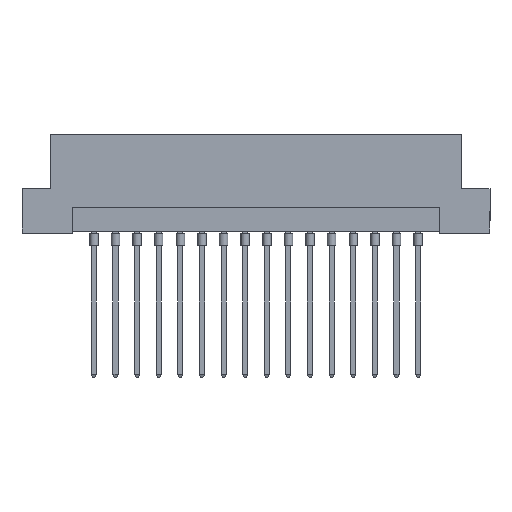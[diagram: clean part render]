
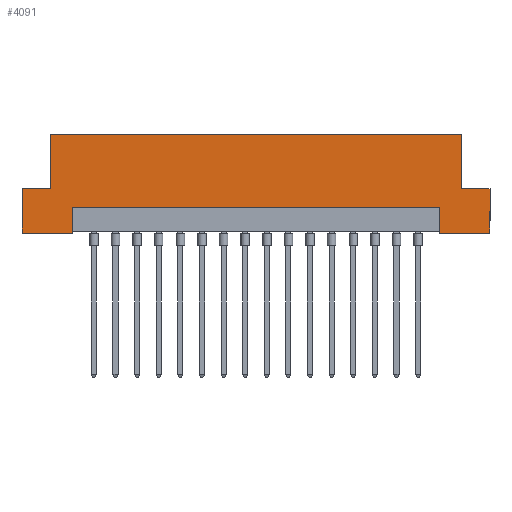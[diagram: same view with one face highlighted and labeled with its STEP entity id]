
A CAD part, front view. The second image highlights one B-rep face of the part: STEP entity #4091.
In plain terms, the highlighted planar face has unit normal (0, -1, 0).
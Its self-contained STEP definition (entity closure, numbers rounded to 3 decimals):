
#2 = CARTESIAN_POINT ( 'NONE',  ( -21.6, -4.3, 3. ) ) ;
#103 = PLANE ( 'NONE',  #130 ) ;
#130 = AXIS2_PLACEMENT_3D ( 'NONE', #2309, #6668, #549 ) ;
#206 = VECTOR ( 'NONE', #3185, 1000. ) ;
#326 = DIRECTION ( 'NONE',  ( 0., 0., -1. ) ) ;
#549 = DIRECTION ( 'NONE',  ( -1., 0., 0. ) ) ;
#552 = LINE ( 'NONE', #2, #6739 ) ;
#557 = CARTESIAN_POINT ( 'NONE',  ( -27.5, -4.3, 5.2 ) ) ;
#579 = ORIENTED_EDGE ( 'NONE', *, *, #829, .F. ) ;
#670 = VERTEX_POINT ( 'NONE', #2685 ) ;
#740 = ORIENTED_EDGE ( 'NONE', *, *, #3811, .T. ) ;
#774 = ORIENTED_EDGE ( 'NONE', *, *, #5839, .T. ) ;
#792 = VERTEX_POINT ( 'NONE', #2486 ) ;
#829 = EDGE_CURVE ( 'NONE', #3084, #792, #4149, .T. ) ;
#835 = CARTESIAN_POINT ( 'NONE',  ( 27.5, -4.3, 11.6 ) ) ;
#889 = ORIENTED_EDGE ( 'NONE', *, *, #3107, .F. ) ;
#1007 = CARTESIAN_POINT ( 'NONE',  ( 24.2, -4.3, 11.6 ) ) ;
#1093 = VECTOR ( 'NONE', #326, 1000. ) ;
#1179 = CARTESIAN_POINT ( 'NONE',  ( -24.2, -4.3, 11.6 ) ) ;
#1221 = VERTEX_POINT ( 'NONE', #3949 ) ;
#1321 = EDGE_CURVE ( 'NONE', #4698, #2654, #3849, .T. ) ;
#1358 = EDGE_CURVE ( 'NONE', #4435, #5169, #5413, .T. ) ;
#1400 = ORIENTED_EDGE ( 'NONE', *, *, #6419, .F. ) ;
#1485 = LINE ( 'NONE', #1559, #2424 ) ;
#1507 = CARTESIAN_POINT ( 'NONE',  ( 24.2, -4.3, 5.2 ) ) ;
#1559 = CARTESIAN_POINT ( 'NONE',  ( -24.2, -4.3, 5.2 ) ) ;
#1581 = ORIENTED_EDGE ( 'NONE', *, *, #1358, .T. ) ;
#1678 = VECTOR ( 'NONE', #7025, 1000. ) ;
#1768 = ORIENTED_EDGE ( 'NONE', *, *, #1321, .T. ) ;
#1873 = VECTOR ( 'NONE', #6663, 1000. ) ;
#1889 = CARTESIAN_POINT ( 'NONE',  ( -27.5, -4.3, 0. ) ) ;
#1924 = VERTEX_POINT ( 'NONE', #2289 ) ;
#1949 = EDGE_LOOP ( 'NONE', ( #774, #889, #740, #579, #3532, #1768, #5623, #6495, #3735, #1581, #3248, #1400 ) ) ;
#2173 = CARTESIAN_POINT ( 'NONE',  ( 27.5, -4.3, 0. ) ) ;
#2289 = CARTESIAN_POINT ( 'NONE',  ( 21.6, -4.3, 0. ) ) ;
#2309 = CARTESIAN_POINT ( 'NONE',  ( 27.5, -4.3, 11.6 ) ) ;
#2424 = VECTOR ( 'NONE', #5394, 1000. ) ;
#2486 = CARTESIAN_POINT ( 'NONE',  ( 27.5, -4.3, 0. ) ) ;
#2616 = CARTESIAN_POINT ( 'NONE',  ( 27.5, -4.3, 5.2 ) ) ;
#2654 = VERTEX_POINT ( 'NONE', #1007 ) ;
#2670 = EDGE_CURVE ( 'NONE', #5807, #6868, #1485, .T. ) ;
#2685 = CARTESIAN_POINT ( 'NONE',  ( 21.6, -4.3, 3. ) ) ;
#2849 = CARTESIAN_POINT ( 'NONE',  ( -21.6, -4.3, 0.2 ) ) ;
#2886 = LINE ( 'NONE', #6812, #6394 ) ;
#2916 = CARTESIAN_POINT ( 'NONE',  ( 24.2, -4.3, 5.2 ) ) ;
#2957 = DIRECTION ( 'NONE',  ( 1., 0., 0. ) ) ;
#3084 = VERTEX_POINT ( 'NONE', #2616 ) ;
#3107 = EDGE_CURVE ( 'NONE', #1924, #670, #3690, .T. ) ;
#3131 = LINE ( 'NONE', #4185, #4292 ) ;
#3185 = DIRECTION ( 'NONE',  ( 0., 0., 1. ) ) ;
#3192 = DIRECTION ( 'NONE',  ( 0., 0., 1. ) ) ;
#3229 = VECTOR ( 'NONE', #3428, 1000. ) ;
#3248 = ORIENTED_EDGE ( 'NONE', *, *, #4099, .T. ) ;
#3428 = DIRECTION ( 'NONE',  ( 1., 0., 0. ) ) ;
#3499 = LINE ( 'NONE', #3564, #7079 ) ;
#3532 = ORIENTED_EDGE ( 'NONE', *, *, #6048, .F. ) ;
#3564 = CARTESIAN_POINT ( 'NONE',  ( 27.5, -4.3, 0. ) ) ;
#3608 = DIRECTION ( 'NONE',  ( 1., 0., 0. ) ) ;
#3643 = EDGE_CURVE ( 'NONE', #4435, #5807, #3837, .T. ) ;
#3690 = LINE ( 'NONE', #5442, #206 ) ;
#3735 = ORIENTED_EDGE ( 'NONE', *, *, #3643, .F. ) ;
#3811 = EDGE_CURVE ( 'NONE', #1924, #792, #3499, .T. ) ;
#3837 = LINE ( 'NONE', #557, #3229 ) ;
#3849 = LINE ( 'NONE', #1507, #5491 ) ;
#3920 = CARTESIAN_POINT ( 'NONE',  ( -21.6, -4.3, 3. ) ) ;
#3949 = CARTESIAN_POINT ( 'NONE',  ( -21.6, -4.3, 0. ) ) ;
#4091 = ADVANCED_FACE ( 'NONE', ( #4473 ), #103, .F. ) ;
#4099 = EDGE_CURVE ( 'NONE', #5169, #1221, #6057, .T. ) ;
#4149 = LINE ( 'NONE', #835, #1093 ) ;
#4185 = CARTESIAN_POINT ( 'NONE',  ( 27.5, -4.3, 11.6 ) ) ;
#4292 = VECTOR ( 'NONE', #4778, 1000. ) ;
#4435 = VERTEX_POINT ( 'NONE', #6444 ) ;
#4448 = CARTESIAN_POINT ( 'NONE',  ( -24.2, -4.3, 5.2 ) ) ;
#4473 = FACE_OUTER_BOUND ( 'NONE', #1949, .T. ) ;
#4529 = VERTEX_POINT ( 'NONE', #3920 ) ;
#4698 = VERTEX_POINT ( 'NONE', #2916 ) ;
#4749 = VECTOR ( 'NONE', #5534, 1000. ) ;
#4778 = DIRECTION ( 'NONE',  ( 1., 0., 0. ) ) ;
#5169 = VERTEX_POINT ( 'NONE', #1889 ) ;
#5394 = DIRECTION ( 'NONE',  ( 0., 0., 1. ) ) ;
#5413 = LINE ( 'NONE', #5946, #1678 ) ;
#5442 = CARTESIAN_POINT ( 'NONE',  ( 21.6, -4.3, 0.2 ) ) ;
#5491 = VECTOR ( 'NONE', #3192, 1000. ) ;
#5534 = DIRECTION ( 'NONE',  ( 1., 0., 0. ) ) ;
#5540 = DIRECTION ( 'NONE',  ( 1., 0., 0. ) ) ;
#5623 = ORIENTED_EDGE ( 'NONE', *, *, #6102, .F. ) ;
#5807 = VERTEX_POINT ( 'NONE', #4448 ) ;
#5839 = EDGE_CURVE ( 'NONE', #4529, #670, #552, .T. ) ;
#5946 = CARTESIAN_POINT ( 'NONE',  ( -27.5, -4.3, 11.6 ) ) ;
#6048 = EDGE_CURVE ( 'NONE', #4698, #3084, #2886, .T. ) ;
#6057 = LINE ( 'NONE', #2173, #4749 ) ;
#6102 = EDGE_CURVE ( 'NONE', #6868, #2654, #3131, .T. ) ;
#6163 = LINE ( 'NONE', #2849, #1873 ) ;
#6394 = VECTOR ( 'NONE', #2957, 1000. ) ;
#6419 = EDGE_CURVE ( 'NONE', #4529, #1221, #6163, .T. ) ;
#6444 = CARTESIAN_POINT ( 'NONE',  ( -27.5, -4.3, 5.2 ) ) ;
#6495 = ORIENTED_EDGE ( 'NONE', *, *, #2670, .F. ) ;
#6663 = DIRECTION ( 'NONE',  ( 0., 0., -1. ) ) ;
#6668 = DIRECTION ( 'NONE',  ( 0., 1., 0. ) ) ;
#6739 = VECTOR ( 'NONE', #5540, 1000. ) ;
#6812 = CARTESIAN_POINT ( 'NONE',  ( 27.5, -4.3, 5.2 ) ) ;
#6868 = VERTEX_POINT ( 'NONE', #1179 ) ;
#7025 = DIRECTION ( 'NONE',  ( 0., 0., -1. ) ) ;
#7079 = VECTOR ( 'NONE', #3608, 1000. ) ;
